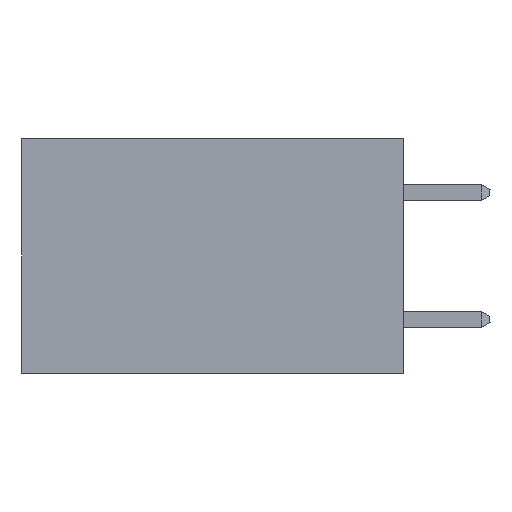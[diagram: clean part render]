
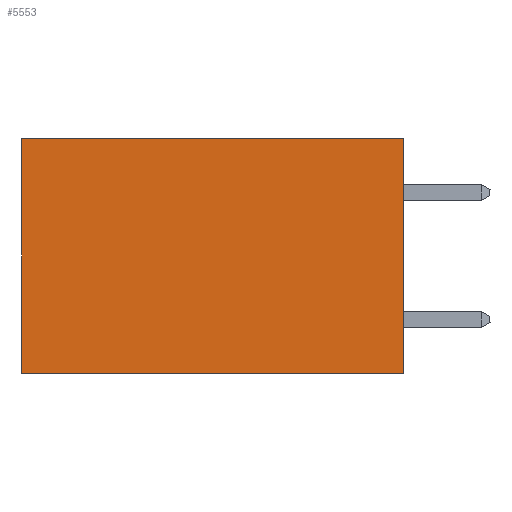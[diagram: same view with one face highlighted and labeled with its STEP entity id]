
A CAD part, left-side view. The second image highlights one B-rep face of the part: STEP entity #5553.
In plain terms, the highlighted planar face has unit normal (-1, 0, 0).
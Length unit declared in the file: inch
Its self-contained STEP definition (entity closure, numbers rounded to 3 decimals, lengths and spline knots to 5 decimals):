
#348 = CARTESIAN_POINT ( 'NONE',  ( 0.2875, 0.6, -0.37 ) ) ;
#1131 = DIRECTION ( 'NONE',  ( 0., 0., -1. ) ) ;
#2124 = DIRECTION ( 'NONE',  ( 0., 1., 0. ) ) ;
#2247 = EDGE_CURVE ( 'NONE', #15745, #16114, #29053, .T. ) ;
#2547 = DIRECTION ( 'NONE',  ( 0., 0., -1. ) ) ;
#3659 = CARTESIAN_POINT ( 'NONE',  ( 0.2875, 0.6, 0. ) ) ;
#4441 = CARTESIAN_POINT ( 'NONE',  ( 0.2875, 0.6, 0. ) ) ;
#4526 = CARTESIAN_POINT ( 'NONE',  ( 0.2875, 0., 0. ) ) ;
#5214 = PLANE ( 'NONE',  #14184 ) ;
#5553 = ADVANCED_FACE ( 'NONE', ( #12808 ), #5214, .F. ) ;
#5870 = ORIENTED_EDGE ( 'NONE', *, *, #2247, .T. ) ;
#7705 = EDGE_CURVE ( 'NONE', #24415, #15745, #22750, .T. ) ;
#7712 = DIRECTION ( 'NONE',  ( 0., 1., 0. ) ) ;
#11416 = LINE ( 'NONE', #13375, #28200 ) ;
#12808 = FACE_OUTER_BOUND ( 'NONE', #22399, .T. ) ;
#13375 = CARTESIAN_POINT ( 'NONE',  ( 0.2875, 0., -0.37 ) ) ;
#13382 = CARTESIAN_POINT ( 'NONE',  ( 0.2875, 0., -0.37 ) ) ;
#13435 = EDGE_CURVE ( 'NONE', #22485, #16114, #11416, .T. ) ;
#13458 = VECTOR ( 'NONE', #1131, 39.37008 ) ;
#14184 = AXIS2_PLACEMENT_3D ( 'NONE', #17093, #19917, #25573 ) ;
#14664 = CARTESIAN_POINT ( 'NONE',  ( 0.2875, 0., 0. ) ) ;
#15138 = EDGE_CURVE ( 'NONE', #24415, #22485, #18829, .T. ) ;
#15745 = VERTEX_POINT ( 'NONE', #3659 ) ;
#16114 = VERTEX_POINT ( 'NONE', #348 ) ;
#17093 = CARTESIAN_POINT ( 'NONE',  ( 0.2875, 0., 0. ) ) ;
#18829 = LINE ( 'NONE', #14664, #13458 ) ;
#19917 = DIRECTION ( 'NONE',  ( 1., 0., 0. ) ) ;
#20323 = ORIENTED_EDGE ( 'NONE', *, *, #13435, .F. ) ;
#21485 = ORIENTED_EDGE ( 'NONE', *, *, #15138, .F. ) ;
#22286 = ORIENTED_EDGE ( 'NONE', *, *, #7705, .T. ) ;
#22399 = EDGE_LOOP ( 'NONE', ( #5870, #20323, #21485, #22286 ) ) ;
#22485 = VERTEX_POINT ( 'NONE', #13382 ) ;
#22750 = LINE ( 'NONE', #23615, #28824 ) ;
#22961 = VECTOR ( 'NONE', #2547, 39.37008 ) ;
#23615 = CARTESIAN_POINT ( 'NONE',  ( 0.2875, 0., 0. ) ) ;
#24415 = VERTEX_POINT ( 'NONE', #4526 ) ;
#25573 = DIRECTION ( 'NONE',  ( 0., 0., -1. ) ) ;
#28200 = VECTOR ( 'NONE', #2124, 39.37008 ) ;
#28824 = VECTOR ( 'NONE', #7712, 39.37008 ) ;
#29053 = LINE ( 'NONE', #4441, #22961 ) ;
